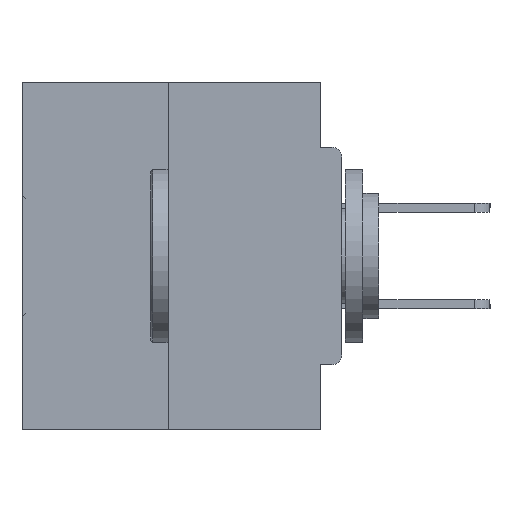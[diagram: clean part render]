
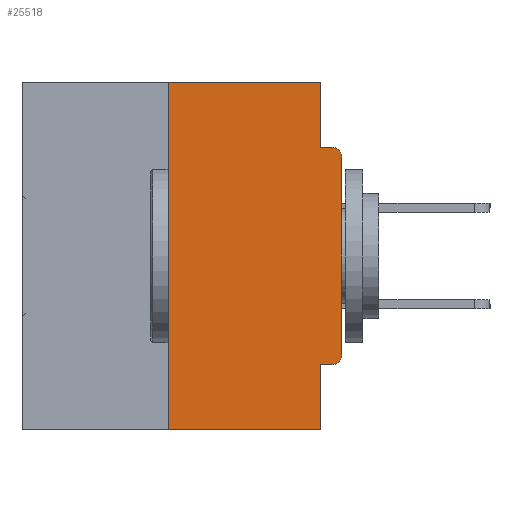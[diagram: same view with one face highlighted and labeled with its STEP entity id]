
A CAD part, left-side view. The second image highlights one B-rep face of the part: STEP entity #25518.
In plain terms, the highlighted planar face has unit normal (-1, 0, 0).
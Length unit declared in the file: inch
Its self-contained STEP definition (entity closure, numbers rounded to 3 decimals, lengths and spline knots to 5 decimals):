
#67 = VECTOR ( 'NONE', #14045, 39.37008 ) ;
#1059 = VERTEX_POINT ( 'NONE', #32845 ) ;
#1190 = CARTESIAN_POINT ( 'NONE',  ( 0., 0.25, -0.5 ) ) ;
#1830 = ORIENTED_EDGE ( 'NONE', *, *, #26705, .F. ) ;
#2302 = CARTESIAN_POINT ( 'NONE',  ( 0., 0.031, -0.0935 ) ) ;
#2565 = LINE ( 'NONE', #19264, #42357 ) ;
#3767 = VERTEX_POINT ( 'NONE', #1190 ) ;
#4301 = CARTESIAN_POINT ( 'NONE',  ( 0., 0.031, 0. ) ) ;
#4590 = DIRECTION ( 'NONE',  ( 1., 0., 0. ) ) ;
#5156 = EDGE_CURVE ( 'NONE', #18787, #36972, #27592, .T. ) ;
#5269 = ORIENTED_EDGE ( 'NONE', *, *, #39770, .F. ) ;
#5289 = LINE ( 'NONE', #5359, #40452 ) ;
#5359 = CARTESIAN_POINT ( 'NONE',  ( 0., 0., -0.4065 ) ) ;
#5622 = DIRECTION ( 'NONE',  ( -1., 0., 0. ) ) ;
#6061 = ORIENTED_EDGE ( 'NONE', *, *, #28463, .F. ) ;
#6268 = EDGE_CURVE ( 'NONE', #7803, #36972, #19953, .T. ) ;
#6289 = ORIENTED_EDGE ( 'NONE', *, *, #28034, .T. ) ;
#6927 = CARTESIAN_POINT ( 'NONE',  ( 0., 0.015, -0.4065 ) ) ;
#7803 = VERTEX_POINT ( 'NONE', #2302 ) ;
#8047 = EDGE_CURVE ( 'NONE', #37876, #39814, #15485, .T. ) ;
#8051 = FACE_OUTER_BOUND ( 'NONE', #42623, .T. ) ;
#8104 = VECTOR ( 'NONE', #23839, 39.37008 ) ;
#8489 = CARTESIAN_POINT ( 'NONE',  ( 0., 0.031, -0.5 ) ) ;
#9352 = ORIENTED_EDGE ( 'NONE', *, *, #27054, .F. ) ;
#9709 = LINE ( 'NONE', #37911, #8104 ) ;
#13346 = VECTOR ( 'NONE', #22343, 39.37008 ) ;
#13900 = VERTEX_POINT ( 'NONE', #4301 ) ;
#14045 = DIRECTION ( 'NONE',  ( 0., -1., 0. ) ) ;
#14323 = CARTESIAN_POINT ( 'NONE',  ( 0., 0.015, -0.0935 ) ) ;
#14680 = ORIENTED_EDGE ( 'NONE', *, *, #35712, .T. ) ;
#15383 = DIRECTION ( 'NONE',  ( 0., -1., 0. ) ) ;
#15452 = CARTESIAN_POINT ( 'NONE',  ( 0., 0.015, -0.1085 ) ) ;
#15485 = CIRCLE ( 'NONE', #29140, 0.015 ) ;
#16752 = CARTESIAN_POINT ( 'NONE',  ( 0., 0., -0.0935 ) ) ;
#17670 = DIRECTION ( 'NONE',  ( 0., 0., -1. ) ) ;
#18123 = LINE ( 'NONE', #18990, #37426 ) ;
#18756 = DIRECTION ( 'NONE',  ( 0., 0., -1. ) ) ;
#18764 = LINE ( 'NONE', #18875, #13346 ) ;
#18787 = VERTEX_POINT ( 'NONE', #32950 ) ;
#18875 = CARTESIAN_POINT ( 'NONE',  ( 0., 0.031, -0.5 ) ) ;
#18990 = CARTESIAN_POINT ( 'NONE',  ( 0., 0.46, -0.5 ) ) ;
#19264 = CARTESIAN_POINT ( 'NONE',  ( 0., 0.25, 0. ) ) ;
#19953 = LINE ( 'NONE', #16752, #67 ) ;
#22343 = DIRECTION ( 'NONE',  ( 0., 0., -1. ) ) ;
#23061 = DIRECTION ( 'NONE',  ( 0., -1., 0. ) ) ;
#23311 = LINE ( 'NONE', #26349, #29791 ) ;
#23408 = VERTEX_POINT ( 'NONE', #43315 ) ;
#23839 = DIRECTION ( 'NONE',  ( 0., 0., 1. ) ) ;
#24241 = ORIENTED_EDGE ( 'NONE', *, *, #32182, .F. ) ;
#24855 = CARTESIAN_POINT ( 'NONE',  ( 0., 0.015, -0.3915 ) ) ;
#24994 = DIRECTION ( 'NONE',  ( -1., 0., 0. ) ) ;
#25518 = ADVANCED_FACE ( 'NONE', ( #8051 ), #29259, .F. ) ;
#25541 = VERTEX_POINT ( 'NONE', #8489 ) ;
#26258 = ORIENTED_EDGE ( 'NONE', *, *, #5156, .T. ) ;
#26349 = CARTESIAN_POINT ( 'NONE',  ( 0., 0.46, 0. ) ) ;
#26705 = EDGE_CURVE ( 'NONE', #37876, #1059, #5289, .T. ) ;
#27054 = EDGE_CURVE ( 'NONE', #1059, #25541, #18764, .T. ) ;
#27592 = CIRCLE ( 'NONE', #38272, 0.015 ) ;
#28034 = EDGE_CURVE ( 'NONE', #3767, #25541, #18123, .T. ) ;
#28134 = ORIENTED_EDGE ( 'NONE', *, *, #6268, .F. ) ;
#28463 = EDGE_CURVE ( 'NONE', #13900, #7803, #30986, .T. ) ;
#28908 = DIRECTION ( 'NONE',  ( 0., 0., 1. ) ) ;
#29140 = AXIS2_PLACEMENT_3D ( 'NONE', #24855, #24994, #17670 ) ;
#29259 = PLANE ( 'NONE',  #38016 ) ;
#29743 = DIRECTION ( 'NONE',  ( 0., 0., -1. ) ) ;
#29791 = VECTOR ( 'NONE', #23061, 39.37008 ) ;
#30986 = LINE ( 'NONE', #35474, #36847 ) ;
#32182 = EDGE_CURVE ( 'NONE', #3767, #23408, #2565, .T. ) ;
#32845 = CARTESIAN_POINT ( 'NONE',  ( 0., 0.031, -0.4065 ) ) ;
#32891 = DIRECTION ( 'NONE',  ( 0., 1., 0. ) ) ;
#32950 = CARTESIAN_POINT ( 'NONE',  ( 0., 0., -0.1085 ) ) ;
#33107 = CARTESIAN_POINT ( 'NONE',  ( 0., 0., -0.3915 ) ) ;
#33644 = ORIENTED_EDGE ( 'NONE', *, *, #8047, .T. ) ;
#35474 = CARTESIAN_POINT ( 'NONE',  ( 0., 0.031, 0. ) ) ;
#35712 = EDGE_CURVE ( 'NONE', #39814, #18787, #9709, .T. ) ;
#36847 = VECTOR ( 'NONE', #42320, 39.37008 ) ;
#36972 = VERTEX_POINT ( 'NONE', #14323 ) ;
#37426 = VECTOR ( 'NONE', #15383, 39.37008 ) ;
#37876 = VERTEX_POINT ( 'NONE', #6927 ) ;
#37911 = CARTESIAN_POINT ( 'NONE',  ( 0., 0., 0. ) ) ;
#38016 = AXIS2_PLACEMENT_3D ( 'NONE', #39294, #4590, #18756 ) ;
#38272 = AXIS2_PLACEMENT_3D ( 'NONE', #15452, #5622, #29743 ) ;
#39294 = CARTESIAN_POINT ( 'NONE',  ( 0., 0.46, 0. ) ) ;
#39770 = EDGE_CURVE ( 'NONE', #23408, #13900, #23311, .T. ) ;
#39814 = VERTEX_POINT ( 'NONE', #33107 ) ;
#40452 = VECTOR ( 'NONE', #32891, 39.37008 ) ;
#42320 = DIRECTION ( 'NONE',  ( 0., 0., -1. ) ) ;
#42357 = VECTOR ( 'NONE', #28908, 39.37008 ) ;
#42623 = EDGE_LOOP ( 'NONE', ( #5269, #24241, #6289, #9352, #1830, #33644, #14680, #26258, #28134, #6061 ) ) ;
#43315 = CARTESIAN_POINT ( 'NONE',  ( 0., 0.25, 0. ) ) ;
